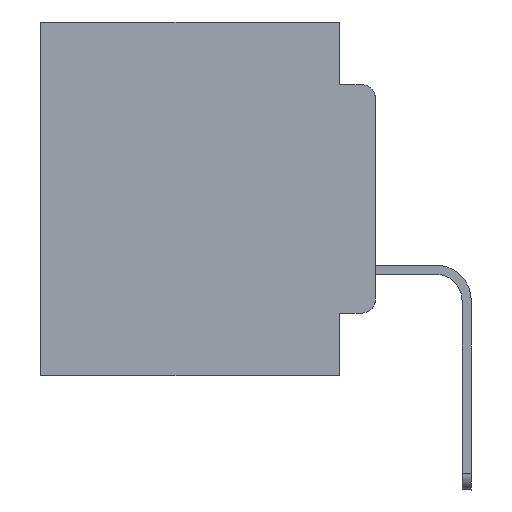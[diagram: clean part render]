
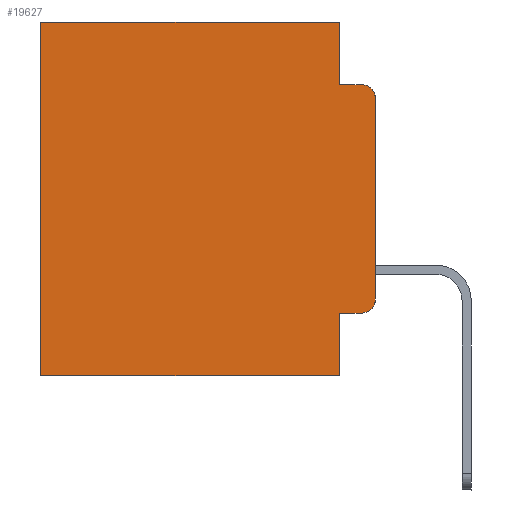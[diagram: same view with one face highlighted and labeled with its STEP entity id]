
A CAD part, left-side view. The second image highlights one B-rep face of the part: STEP entity #19627.
In plain terms, the highlighted planar face has unit normal (-1, 0, 0).
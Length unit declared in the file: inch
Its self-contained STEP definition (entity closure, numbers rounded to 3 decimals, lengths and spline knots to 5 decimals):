
#47 = PLANE ( 'NONE',  #2091 ) ;
#452 = AXIS2_PLACEMENT_3D ( 'NONE', #15763, #25294, #21378 ) ;
#489 = CARTESIAN_POINT ( 'NONE',  ( 0.298, 0., 0. ) ) ;
#823 = DIRECTION ( 'NONE',  ( -1., 0., 0. ) ) ;
#933 = DIRECTION ( 'NONE',  ( 0., -1., 0. ) ) ;
#1065 = DIRECTION ( 'NONE',  ( 0., 0., -1. ) ) ;
#1872 = DIRECTION ( 'NONE',  ( 0., 0., -1. ) ) ;
#2091 = AXIS2_PLACEMENT_3D ( 'NONE', #9749, #19745, #1872 ) ;
#2555 = VERTEX_POINT ( 'NONE', #10972 ) ;
#3013 = VERTEX_POINT ( 'NONE', #11992 ) ;
#3422 = VERTEX_POINT ( 'NONE', #10794 ) ;
#3896 = FACE_OUTER_BOUND ( 'NONE', #8800, .T. ) ;
#4086 = ORIENTED_EDGE ( 'NONE', *, *, #15659, .T. ) ;
#4486 = LINE ( 'NONE', #18769, #15820 ) ;
#4560 = EDGE_CURVE ( 'NONE', #3013, #24438, #18446, .T. ) ;
#4821 = ORIENTED_EDGE ( 'NONE', *, *, #19941, .F. ) ;
#5500 = DIRECTION ( 'NONE',  ( 0., 0., -1. ) ) ;
#6283 = CARTESIAN_POINT ( 'NONE',  ( 0.298, 0.473, 0. ) ) ;
#6725 = VERTEX_POINT ( 'NONE', #18436 ) ;
#6928 = LINE ( 'NONE', #23333, #10893 ) ;
#8050 = VERTEX_POINT ( 'NONE', #19227 ) ;
#8224 = VECTOR ( 'NONE', #24289, 39.37008 ) ;
#8405 = ORIENTED_EDGE ( 'NONE', *, *, #4560, .F. ) ;
#8800 = EDGE_LOOP ( 'NONE', ( #4821, #11634, #25479, #21106, #12111, #24911, #8405, #12427, #4086, #20150 ) ) ;
#8989 = VERTEX_POINT ( 'NONE', #17864 ) ;
#9613 = CARTESIAN_POINT ( 'NONE',  ( 0.298, 0., -0.5 ) ) ;
#9749 = CARTESIAN_POINT ( 'NONE',  ( 0.298, 0., 0. ) ) ;
#10612 = EDGE_CURVE ( 'NONE', #8989, #2555, #24395, .T. ) ;
#10716 = VECTOR ( 'NONE', #13566, 39.37008 ) ;
#10794 = CARTESIAN_POINT ( 'NONE',  ( 0.298, 0.02, -0.0885 ) ) ;
#10893 = VECTOR ( 'NONE', #5500, 39.37008 ) ;
#10972 = CARTESIAN_POINT ( 'NONE',  ( 0.298, 0., -0.3915 ) ) ;
#10989 = AXIS2_PLACEMENT_3D ( 'NONE', #24606, #823, #12737 ) ;
#11168 = CARTESIAN_POINT ( 'NONE',  ( 0.298, 0.473, -0.5 ) ) ;
#11192 = VECTOR ( 'NONE', #11542, 39.37008 ) ;
#11264 = CARTESIAN_POINT ( 'NONE',  ( 0.298, 0.051, 0. ) ) ;
#11380 = VERTEX_POINT ( 'NONE', #6283 ) ;
#11542 = DIRECTION ( 'NONE',  ( 0., -1., 0. ) ) ;
#11634 = ORIENTED_EDGE ( 'NONE', *, *, #14310, .T. ) ;
#11969 = CIRCLE ( 'NONE', #10989, 0.02 ) ;
#11992 = CARTESIAN_POINT ( 'NONE',  ( 0.298, 0.051, -0.5 ) ) ;
#12111 = ORIENTED_EDGE ( 'NONE', *, *, #17396, .T. ) ;
#12173 = VECTOR ( 'NONE', #933, 39.37008 ) ;
#12427 = ORIENTED_EDGE ( 'NONE', *, *, #25279, .F. ) ;
#12737 = DIRECTION ( 'NONE',  ( 0., 0., -1. ) ) ;
#12785 = LINE ( 'NONE', #14585, #12173 ) ;
#13416 = VERTEX_POINT ( 'NONE', #17641 ) ;
#13450 = LINE ( 'NONE', #489, #8224 ) ;
#13566 = DIRECTION ( 'NONE',  ( 0., 1., 0. ) ) ;
#13675 = LINE ( 'NONE', #23666, #11192 ) ;
#14310 = EDGE_CURVE ( 'NONE', #15048, #3422, #11969, .T. ) ;
#14514 = EDGE_CURVE ( 'NONE', #13416, #6725, #22469, .T. ) ;
#14585 = CARTESIAN_POINT ( 'NONE',  ( 0.298, 0.051, -0.4115 ) ) ;
#15048 = VERTEX_POINT ( 'NONE', #24584 ) ;
#15659 = EDGE_CURVE ( 'NONE', #8050, #8989, #12785, .T. ) ;
#15763 = CARTESIAN_POINT ( 'NONE',  ( 0.298, 0.02, -0.3915 ) ) ;
#15820 = VECTOR ( 'NONE', #1065, 39.37008 ) ;
#16182 = EDGE_CURVE ( 'NONE', #11380, #24438, #6928, .T. ) ;
#17396 = EDGE_CURVE ( 'NONE', #13416, #11380, #13450, .T. ) ;
#17641 = CARTESIAN_POINT ( 'NONE',  ( 0.298, 0.051, 0. ) ) ;
#17810 = VECTOR ( 'NONE', #25117, 39.37008 ) ;
#17864 = CARTESIAN_POINT ( 'NONE',  ( 0.298, 0.02, -0.4115 ) ) ;
#18436 = CARTESIAN_POINT ( 'NONE',  ( 0.298, 0.051, -0.0885 ) ) ;
#18446 = LINE ( 'NONE', #9613, #10716 ) ;
#18744 = DIRECTION ( 'NONE',  ( 0., 0., -1. ) ) ;
#18769 = CARTESIAN_POINT ( 'NONE',  ( 0.298, 0., 0. ) ) ;
#19020 = VECTOR ( 'NONE', #18744, 39.37008 ) ;
#19227 = CARTESIAN_POINT ( 'NONE',  ( 0.298, 0.051, -0.4115 ) ) ;
#19584 = EDGE_CURVE ( 'NONE', #6725, #3422, #13675, .T. ) ;
#19627 = ADVANCED_FACE ( 'NONE', ( #3896 ), #47, .F. ) ;
#19745 = DIRECTION ( 'NONE',  ( 1., 0., 0. ) ) ;
#19941 = EDGE_CURVE ( 'NONE', #15048, #2555, #4486, .T. ) ;
#20150 = ORIENTED_EDGE ( 'NONE', *, *, #10612, .T. ) ;
#21106 = ORIENTED_EDGE ( 'NONE', *, *, #14514, .F. ) ;
#21378 = DIRECTION ( 'NONE',  ( 0., 0., -1. ) ) ;
#22469 = LINE ( 'NONE', #11264, #17810 ) ;
#23333 = CARTESIAN_POINT ( 'NONE',  ( 0.298, 0.473, 0. ) ) ;
#23666 = CARTESIAN_POINT ( 'NONE',  ( 0.298, 0.051, -0.0885 ) ) ;
#24289 = DIRECTION ( 'NONE',  ( 0., 1., 0. ) ) ;
#24395 = CIRCLE ( 'NONE', #452, 0.02 ) ;
#24438 = VERTEX_POINT ( 'NONE', #11168 ) ;
#24496 = CARTESIAN_POINT ( 'NONE',  ( 0.298, 0.051, 0. ) ) ;
#24584 = CARTESIAN_POINT ( 'NONE',  ( 0.298, 0., -0.1085 ) ) ;
#24606 = CARTESIAN_POINT ( 'NONE',  ( 0.298, 0.02, -0.1085 ) ) ;
#24630 = LINE ( 'NONE', #24496, #19020 ) ;
#24911 = ORIENTED_EDGE ( 'NONE', *, *, #16182, .T. ) ;
#25117 = DIRECTION ( 'NONE',  ( 0., 0., -1. ) ) ;
#25279 = EDGE_CURVE ( 'NONE', #8050, #3013, #24630, .T. ) ;
#25294 = DIRECTION ( 'NONE',  ( -1., 0., 0. ) ) ;
#25479 = ORIENTED_EDGE ( 'NONE', *, *, #19584, .F. ) ;
